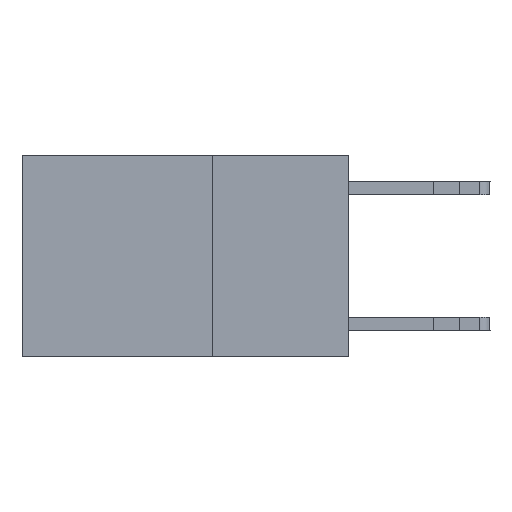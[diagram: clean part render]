
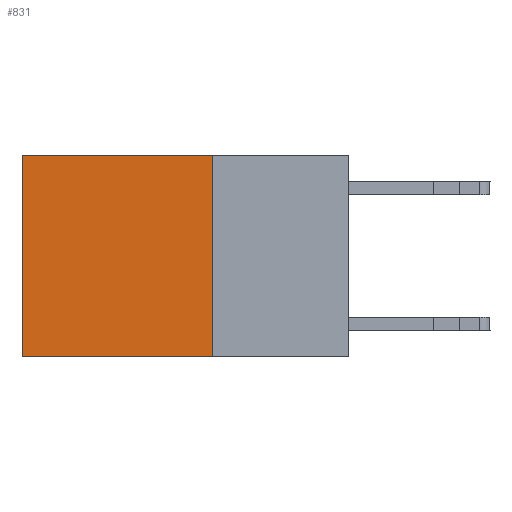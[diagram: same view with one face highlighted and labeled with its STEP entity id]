
A CAD part, left-side view. The second image highlights one B-rep face of the part: STEP entity #831.
In plain terms, the highlighted planar face has unit normal (-1, 0, 0).
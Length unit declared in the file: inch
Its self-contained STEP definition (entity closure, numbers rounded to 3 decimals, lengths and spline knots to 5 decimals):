
#262 = CARTESIAN_POINT ( 'NONE',  ( 0.2625, 0.25, -0.37 ) ) ;
#272 = EDGE_LOOP ( 'NONE', ( #5554, #11058, #607, #9853 ) ) ;
#280 = CARTESIAN_POINT ( 'NONE',  ( 0.2625, 0.25, 0. ) ) ;
#607 = ORIENTED_EDGE ( 'NONE', *, *, #10999, .F. ) ;
#831 = ADVANCED_FACE ( 'NONE', ( #2375 ), #5596, .F. ) ;
#1601 = VERTEX_POINT ( 'NONE', #4631 ) ;
#2375 = FACE_OUTER_BOUND ( 'NONE', #272, .T. ) ;
#2858 = EDGE_CURVE ( 'NONE', #3028, #1601, #3538, .T. ) ;
#3028 = VERTEX_POINT ( 'NONE', #9113 ) ;
#3231 = CARTESIAN_POINT ( 'NONE',  ( 0.2625, 0.25, -0.37 ) ) ;
#3538 = LINE ( 'NONE', #7801, #5894 ) ;
#3588 = LINE ( 'NONE', #7847, #11391 ) ;
#4036 = LINE ( 'NONE', #12843, #5839 ) ;
#4308 = EDGE_CURVE ( 'NONE', #11234, #1601, #12909, .T. ) ;
#4631 = CARTESIAN_POINT ( 'NONE',  ( 0.2625, 0.6, -0.37 ) ) ;
#4879 = VERTEX_POINT ( 'NONE', #13171 ) ;
#5554 = ORIENTED_EDGE ( 'NONE', *, *, #2858, .T. ) ;
#5596 = PLANE ( 'NONE',  #6407 ) ;
#5839 = VECTOR ( 'NONE', #8371, 39.37008 ) ;
#5894 = VECTOR ( 'NONE', #6830, 39.37008 ) ;
#6407 = AXIS2_PLACEMENT_3D ( 'NONE', #280, #8794, #13071 ) ;
#6830 = DIRECTION ( 'NONE',  ( 0., 0., -1. ) ) ;
#7470 = DIRECTION ( 'NONE',  ( 0., 1., 0. ) ) ;
#7801 = CARTESIAN_POINT ( 'NONE',  ( 0.2625, 0.6, 0. ) ) ;
#7847 = CARTESIAN_POINT ( 'NONE',  ( 0.2625, 0.25, 0. ) ) ;
#8371 = DIRECTION ( 'NONE',  ( 0., 1., 0. ) ) ;
#8794 = DIRECTION ( 'NONE',  ( 1., 0., 0. ) ) ;
#9113 = CARTESIAN_POINT ( 'NONE',  ( 0.2625, 0.6, 0. ) ) ;
#9853 = ORIENTED_EDGE ( 'NONE', *, *, #13281, .T. ) ;
#10999 = EDGE_CURVE ( 'NONE', #4879, #11234, #3588, .T. ) ;
#11058 = ORIENTED_EDGE ( 'NONE', *, *, #4308, .F. ) ;
#11234 = VERTEX_POINT ( 'NONE', #3231 ) ;
#11391 = VECTOR ( 'NONE', #12103, 39.37008 ) ;
#12103 = DIRECTION ( 'NONE',  ( 0., 0., -1. ) ) ;
#12148 = VECTOR ( 'NONE', #7470, 39.37008 ) ;
#12843 = CARTESIAN_POINT ( 'NONE',  ( 0.2625, 0.25, 0. ) ) ;
#12909 = LINE ( 'NONE', #262, #12148 ) ;
#13071 = DIRECTION ( 'NONE',  ( 0., 0., -1. ) ) ;
#13171 = CARTESIAN_POINT ( 'NONE',  ( 0.2625, 0.25, 0. ) ) ;
#13281 = EDGE_CURVE ( 'NONE', #4879, #3028, #4036, .T. ) ;
